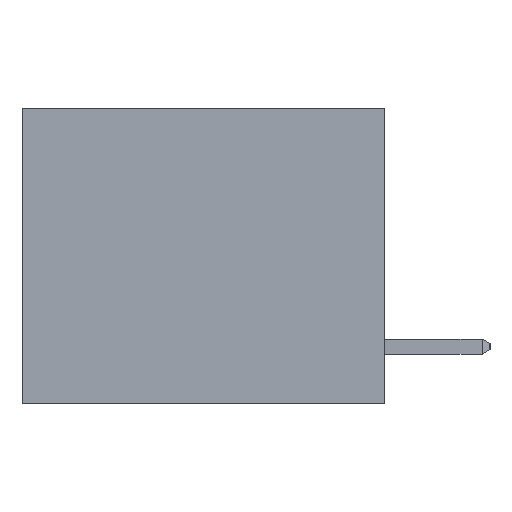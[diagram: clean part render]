
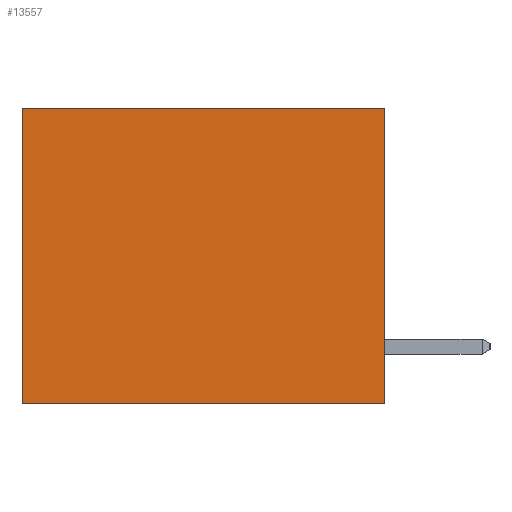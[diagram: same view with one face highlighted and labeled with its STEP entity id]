
A CAD part, left-side view. The second image highlights one B-rep face of the part: STEP entity #13557.
In plain terms, the highlighted planar face has unit normal (-1, 0, 0).
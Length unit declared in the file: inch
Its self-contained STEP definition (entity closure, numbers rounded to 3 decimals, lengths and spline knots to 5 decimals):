
#1212 = CARTESIAN_POINT ( 'NONE',  ( 0.3165, 0., -0.49 ) ) ;
#1705 = EDGE_LOOP ( 'NONE', ( #7308, #18146, #5730, #8153 ) ) ;
#1733 = EDGE_CURVE ( 'NONE', #5589, #6336, #8459, .T. ) ;
#2135 = CARTESIAN_POINT ( 'NONE',  ( 0.3165, 0., -0.49 ) ) ;
#2149 = LINE ( 'NONE', #12981, #9564 ) ;
#2514 = CARTESIAN_POINT ( 'NONE',  ( 0.3165, 0.6, -0.49 ) ) ;
#3266 = CARTESIAN_POINT ( 'NONE',  ( 0.3165, 0., 0. ) ) ;
#4026 = VECTOR ( 'NONE', #21591, 39.37008 ) ;
#4203 = DIRECTION ( 'NONE',  ( 0., 0., -1. ) ) ;
#5589 = VERTEX_POINT ( 'NONE', #3266 ) ;
#5730 = ORIENTED_EDGE ( 'NONE', *, *, #17561, .F. ) ;
#5873 = DIRECTION ( 'NONE',  ( 1., 0., 0. ) ) ;
#6190 = EDGE_CURVE ( 'NONE', #6336, #11692, #19176, .T. ) ;
#6336 = VERTEX_POINT ( 'NONE', #9380 ) ;
#7308 = ORIENTED_EDGE ( 'NONE', *, *, #6190, .T. ) ;
#7772 = PLANE ( 'NONE',  #20945 ) ;
#8118 = EDGE_CURVE ( 'NONE', #17426, #11692, #12892, .T. ) ;
#8153 = ORIENTED_EDGE ( 'NONE', *, *, #1733, .T. ) ;
#8459 = LINE ( 'NONE', #23407, #4026 ) ;
#9380 = CARTESIAN_POINT ( 'NONE',  ( 0.3165, 0.6, 0. ) ) ;
#9564 = VECTOR ( 'NONE', #24377, 39.37008 ) ;
#11172 = FACE_OUTER_BOUND ( 'NONE', #1705, .T. ) ;
#11271 = CARTESIAN_POINT ( 'NONE',  ( 0.3165, 0., -0.49 ) ) ;
#11692 = VERTEX_POINT ( 'NONE', #2514 ) ;
#12892 = LINE ( 'NONE', #11271, #18462 ) ;
#12981 = CARTESIAN_POINT ( 'NONE',  ( 0.3165, 0., -0.49 ) ) ;
#13557 = ADVANCED_FACE ( 'NONE', ( #11172 ), #7772, .F. ) ;
#16214 = VECTOR ( 'NONE', #22374, 39.37008 ) ;
#16477 = CARTESIAN_POINT ( 'NONE',  ( 0.3165, 0.6, -0.49 ) ) ;
#17426 = VERTEX_POINT ( 'NONE', #1212 ) ;
#17561 = EDGE_CURVE ( 'NONE', #5589, #17426, #2149, .T. ) ;
#18146 = ORIENTED_EDGE ( 'NONE', *, *, #8118, .F. ) ;
#18462 = VECTOR ( 'NONE', #20965, 39.37008 ) ;
#19176 = LINE ( 'NONE', #16477, #16214 ) ;
#20945 = AXIS2_PLACEMENT_3D ( 'NONE', #2135, #5873, #4203 ) ;
#20965 = DIRECTION ( 'NONE',  ( 0., 1., 0. ) ) ;
#21591 = DIRECTION ( 'NONE',  ( 0., 1., 0. ) ) ;
#22374 = DIRECTION ( 'NONE',  ( 0., 0., -1. ) ) ;
#23407 = CARTESIAN_POINT ( 'NONE',  ( 0.3165, 0., 0. ) ) ;
#24377 = DIRECTION ( 'NONE',  ( 0., 0., -1. ) ) ;
